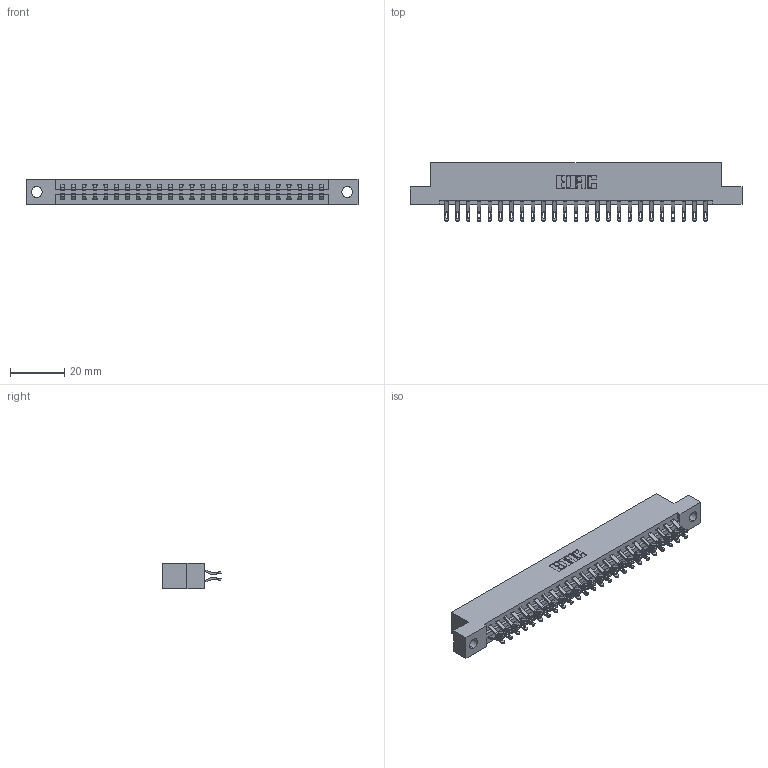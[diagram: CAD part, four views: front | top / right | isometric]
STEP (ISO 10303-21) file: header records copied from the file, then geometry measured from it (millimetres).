
FILE_DESCRIPTION (( 'STEP AP203' ), '1' );
FILE_NAME ('337-050-555-204.STEP', '2019-10-09T16:03:54', ( '' ), ( '' ), 'SwSTEP 2.0', 'SolidWorks 2016', '' );
FILE_SCHEMA (( 'CONFIG_CONTROL_DESIGN' ));
Length unit declared in the file: inch
Products named in the file (3): 337-050-555-204; 345-292-001_555 Tail; 337 Part_Flush Mounting Lugs - 0.156 Dia-TH
Assembly tree (51 placements, depth 2):
  337-050-555-204
    337 Part_Flush Mounting Lugs - 0.156 Dia-TH
    345-292-001_555 Tail  x50
Bounding box: 122.07 x 21.47 x 9.4 mm (x, y, z)
Volume: 12695.8 mm3; surface area: 14531.5 mm2
Topology: 51 solids, 51 shells, 3114 faces, 9761 edges, 6506 vertices
Faces by surface type: plane 1870, cylinder 1244
Entity records: 21911 total; most frequent: CARTESIAN_POINT 3740, ORIENTED_EDGE 3646, DIRECTION 3183, EDGE_CURVE 1823, LINE 1675, VECTOR 1675, VERTEX_POINT 1214, AXIS2_PLACEMENT_3D 754
